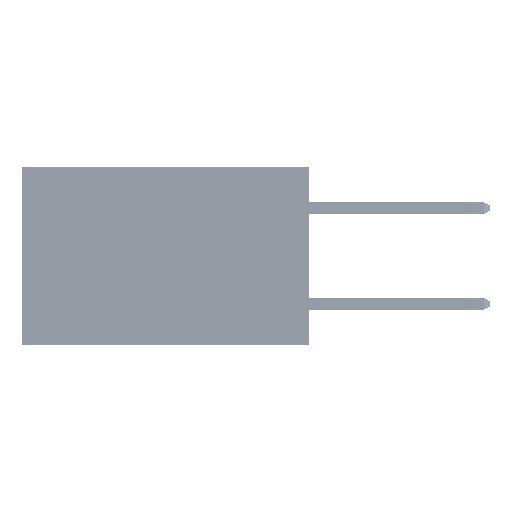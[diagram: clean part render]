
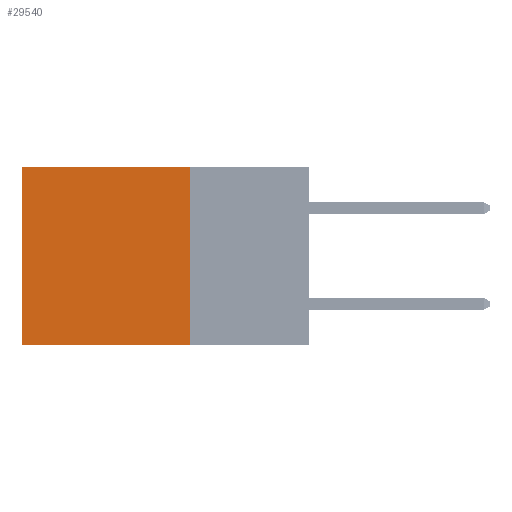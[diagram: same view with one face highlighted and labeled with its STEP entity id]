
A CAD part, left-side view. The second image highlights one B-rep face of the part: STEP entity #29540.
In plain terms, the highlighted planar face has unit normal (-1, 0, 0).
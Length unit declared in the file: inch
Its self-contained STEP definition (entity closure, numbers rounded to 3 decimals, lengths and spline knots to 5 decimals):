
#522 = DIRECTION ( 'NONE',  ( 0., 1., 0. ) ) ;
#1334 = LINE ( 'NONE', #47158, #31915 ) ;
#1445 = CARTESIAN_POINT ( 'NONE',  ( 0.2875, 0.25, 0. ) ) ;
#1543 = LINE ( 'NONE', #50018, #35813 ) ;
#1882 = VERTEX_POINT ( 'NONE', #13025 ) ;
#3962 = EDGE_LOOP ( 'NONE', ( #26255, #11945, #47193, #50105 ) ) ;
#5749 = FACE_OUTER_BOUND ( 'NONE', #3962, .T. ) ;
#6101 = DIRECTION ( 'NONE',  ( 0., 0., -1. ) ) ;
#6294 = CARTESIAN_POINT ( 'NONE',  ( 0.2875, 0.6, 0. ) ) ;
#7434 = CARTESIAN_POINT ( 'NONE',  ( 0.2875, 0.25, 0. ) ) ;
#9948 = LINE ( 'NONE', #6294, #44768 ) ;
#9978 = EDGE_CURVE ( 'NONE', #49377, #1882, #9948, .T. ) ;
#10119 = AXIS2_PLACEMENT_3D ( 'NONE', #1445, #13260, #6101 ) ;
#11945 = ORIENTED_EDGE ( 'NONE', *, *, #37558, .F. ) ;
#13025 = CARTESIAN_POINT ( 'NONE',  ( 0.2875, 0.6, -0.37 ) ) ;
#13260 = DIRECTION ( 'NONE',  ( 1., 0., 0. ) ) ;
#15059 = VECTOR ( 'NONE', #25302, 39.37008 ) ;
#15469 = VERTEX_POINT ( 'NONE', #7434 ) ;
#17309 = CARTESIAN_POINT ( 'NONE',  ( 0.2875, 0.25, 0. ) ) ;
#18536 = DIRECTION ( 'NONE',  ( 0., 0., -1. ) ) ;
#25302 = DIRECTION ( 'NONE',  ( 0., 1., 0. ) ) ;
#25395 = LINE ( 'NONE', #17309, #15059 ) ;
#26255 = ORIENTED_EDGE ( 'NONE', *, *, #9978, .T. ) ;
#28519 = EDGE_CURVE ( 'NONE', #15469, #41903, #1543, .T. ) ;
#29540 = ADVANCED_FACE ( 'NONE', ( #5749 ), #41262, .F. ) ;
#31915 = VECTOR ( 'NONE', #522, 39.37008 ) ;
#31964 = CARTESIAN_POINT ( 'NONE',  ( 0.2875, 0.25, -0.37 ) ) ;
#33942 = EDGE_CURVE ( 'NONE', #15469, #49377, #25395, .T. ) ;
#35813 = VECTOR ( 'NONE', #42733, 39.37008 ) ;
#37558 = EDGE_CURVE ( 'NONE', #41903, #1882, #1334, .T. ) ;
#37713 = CARTESIAN_POINT ( 'NONE',  ( 0.2875, 0.6, 0. ) ) ;
#41262 = PLANE ( 'NONE',  #10119 ) ;
#41903 = VERTEX_POINT ( 'NONE', #31964 ) ;
#42733 = DIRECTION ( 'NONE',  ( 0., 0., -1. ) ) ;
#44768 = VECTOR ( 'NONE', #18536, 39.37008 ) ;
#47158 = CARTESIAN_POINT ( 'NONE',  ( 0.2875, 0.25, -0.37 ) ) ;
#47193 = ORIENTED_EDGE ( 'NONE', *, *, #28519, .F. ) ;
#49377 = VERTEX_POINT ( 'NONE', #37713 ) ;
#50018 = CARTESIAN_POINT ( 'NONE',  ( 0.2875, 0.25, 0. ) ) ;
#50105 = ORIENTED_EDGE ( 'NONE', *, *, #33942, .T. ) ;
